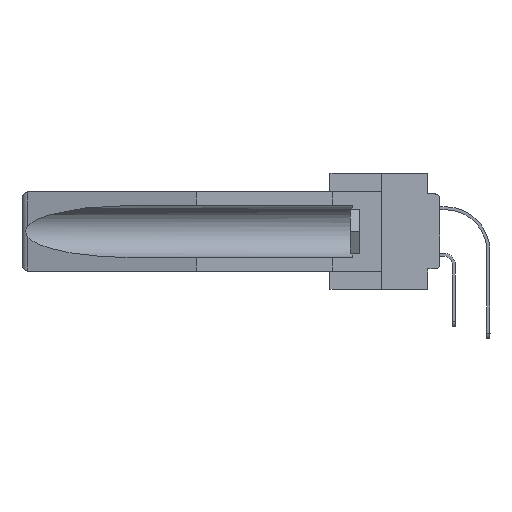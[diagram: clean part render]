
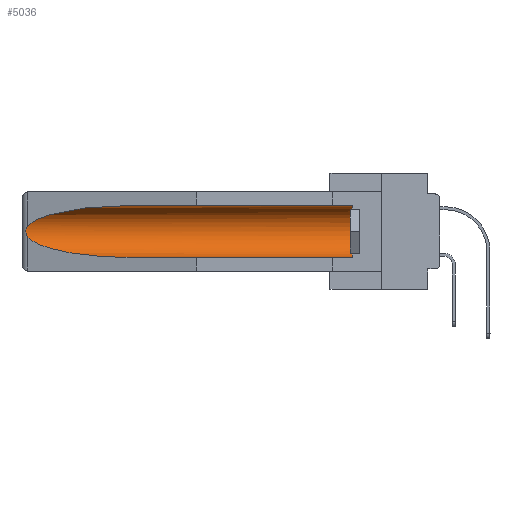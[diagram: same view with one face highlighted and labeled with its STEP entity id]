
A CAD part, left-side view. The second image highlights one B-rep face of the part: STEP entity #5036.
In plain terms, the highlighted cylindrical face has radius 2.857 mm (diameter 5.715 mm), a partial arc.
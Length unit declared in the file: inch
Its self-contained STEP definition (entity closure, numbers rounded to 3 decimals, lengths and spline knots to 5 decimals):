
#527 = CIRCLE ( 'NONE', #28919, 0.1125 ) ;
#611 = EDGE_CURVE ( 'NONE', #28148, #28054, #527, .T. ) ;
#963 = FACE_OUTER_BOUND ( 'NONE', #2200, .T. ) ;
#1455 = CARTESIAN_POINT ( 'NONE',  ( 0.2673, 1.53269, -0.17917 ) ) ;
#1948 = LINE ( 'NONE', #7681, #22371 ) ;
#2200 = EDGE_LOOP ( 'NONE', ( #30819, #31581, #6499, #9714, #12479, #3039 ) ) ;
#2549 = CARTESIAN_POINT ( 'NONE',  ( 0.26537, 1.52718, -0.19328 ) ) ;
#2904 = CARTESIAN_POINT ( 'NONE',  ( 0.25451, 1.48313, -0.09465 ) ) ;
#3039 = ORIENTED_EDGE ( 'NONE', *, *, #29649, .T. ) ;
#4107 = CARTESIAN_POINT ( 'NONE',  ( 0.155, 0.126, -0.284 ) ) ;
#4379 = VERTEX_POINT ( 'NONE', #20845 ) ;
#4663 = CARTESIAN_POINT ( 'NONE',  ( 0.155, 0.126, -0.059 ) ) ;
#5036 = ADVANCED_FACE ( 'NONE', ( #963 ), #13415, .F. ) ;
#5445 = CARTESIAN_POINT ( 'NONE',  ( 0.26537, 1.52718, -0.19328 ) ) ;
#5510 = CARTESIAN_POINT ( 'NONE',  ( 0.155, 1.07973, -0.059 ) ) ;
#5533 = CARTESIAN_POINT ( 'NONE',  ( 0.25451, 1.48313, -0.24835 ) ) ;
#6499 = ORIENTED_EDGE ( 'NONE', *, *, #9204, .T. ) ;
#7393 = CARTESIAN_POINT ( 'NONE',  ( 0.2675, 1.53308, -0.16763 ) ) ;
#7681 = CARTESIAN_POINT ( 'NONE',  ( 0.155, -0.30754, -0.284 ) ) ;
#9204 = EDGE_CURVE ( 'NONE', #37870, #4379, #16370, .T. ) ;
#9714 = ORIENTED_EDGE ( 'NONE', *, *, #23335, .F. ) ;
#10958 = CARTESIAN_POINT ( 'NONE',  ( 0.26537, 1.52718, -0.14972 ) ) ;
#12479 = ORIENTED_EDGE ( 'NONE', *, *, #611, .T. ) ;
#12557 = CARTESIAN_POINT ( 'NONE',  ( 0.26537, 1.52718, -0.14972 ) ) ;
#13068 = EDGE_CURVE ( 'NONE', #22084, #29655, #28942, .T. ) ;
#13267 = B_SPLINE_CURVE_WITH_KNOTS ( 'NONE', 3,
 ( #10958, #34400, #31852, #25753, #7393, #16682, #1455, #28706, #31441, #16884 ),
 .UNSPECIFIED., .F., .F.,
 ( 4, 2, 2, 2, 4 ),
 ( 0., 0.00029, 0.00058, 0.00087, 0.00117 ),
 .UNSPECIFIED. ) ;
#13415 = CYLINDRICAL_SURFACE ( 'NONE', #13519, 0.1125 ) ;
#13519 = AXIS2_PLACEMENT_3D ( 'NONE', #15779, #34482, #25453 ) ;
#15353 = VECTOR ( 'NONE', #37821, 39.37008 ) ;
#15779 = CARTESIAN_POINT ( 'NONE',  ( 0.155, -0.30754, -0.1715 ) ) ;
#16370 =( BOUNDED_CURVE ( )  B_SPLINE_CURVE ( 3, ( #2549, #5533, #17577, #27567 ),
 .UNSPECIFIED., .F., .F. ) 
 B_SPLINE_CURVE_WITH_KNOTS ( ( 4, 4 ),
 ( 0.1948, 1.5708 ),
 .UNSPECIFIED. ) 
 CURVE ( )  GEOMETRIC_REPRESENTATION_ITEM ( )  RATIONAL_B_SPLINE_CURVE ( ( 1., 0.848, 0.848, 1. ) ) 
 REPRESENTATION_ITEM ( '' )  );
#16682 = CARTESIAN_POINT ( 'NONE',  ( 0.2675, 1.53308, -0.17534 ) ) ;
#16884 = CARTESIAN_POINT ( 'NONE',  ( 0.26537, 1.52718, -0.19328 ) ) ;
#16955 = LINE ( 'NONE', #23076, #15353 ) ;
#17577 = CARTESIAN_POINT ( 'NONE',  ( 0.21114, 1.30732, -0.284 ) ) ;
#19797 = EDGE_CURVE ( 'NONE', #29655, #37870, #13267, .T. ) ;
#19952 = DIRECTION ( 'NONE',  ( 0., 1., 0. ) ) ;
#20845 = CARTESIAN_POINT ( 'NONE',  ( 0.155, 1.07973, -0.284 ) ) ;
#22084 = VERTEX_POINT ( 'NONE', #5510 ) ;
#22371 = VECTOR ( 'NONE', #19952, 39.37008 ) ;
#23076 = CARTESIAN_POINT ( 'NONE',  ( 0.155, -0.30754, -0.059 ) ) ;
#23335 = EDGE_CURVE ( 'NONE', #28148, #4379, #1948, .T. ) ;
#24017 = DIRECTION ( 'NONE',  ( 0., 0., 1. ) ) ;
#25453 = DIRECTION ( 'NONE',  ( 0., 0., 1. ) ) ;
#25753 = CARTESIAN_POINT ( 'NONE',  ( 0.2673, 1.5327, -0.16383 ) ) ;
#26979 = CARTESIAN_POINT ( 'NONE',  ( 0.155, 0.126, -0.1715 ) ) ;
#27557 = CARTESIAN_POINT ( 'NONE',  ( 0.21114, 1.30732, -0.059 ) ) ;
#27567 = CARTESIAN_POINT ( 'NONE',  ( 0.155, 1.07973, -0.284 ) ) ;
#28054 = VERTEX_POINT ( 'NONE', #4663 ) ;
#28148 = VERTEX_POINT ( 'NONE', #4107 ) ;
#28706 = CARTESIAN_POINT ( 'NONE',  ( 0.26655, 1.53094, -0.18657 ) ) ;
#28919 = AXIS2_PLACEMENT_3D ( 'NONE', #26979, #38973, #24017 ) ;
#28942 =( BOUNDED_CURVE ( )  B_SPLINE_CURVE ( 3, ( #36406, #27557, #2904, #12557 ),
 .UNSPECIFIED., .F., .F. ) 
 B_SPLINE_CURVE_WITH_KNOTS ( ( 4, 4 ),
 ( 4.71239, 6.08839 ),
 .UNSPECIFIED. ) 
 CURVE ( )  GEOMETRIC_REPRESENTATION_ITEM ( )  RATIONAL_B_SPLINE_CURVE ( ( 1., 0.848, 0.848, 1. ) ) 
 REPRESENTATION_ITEM ( '' )  );
#29649 = EDGE_CURVE ( 'NONE', #28054, #22084, #16955, .T. ) ;
#29655 = VERTEX_POINT ( 'NONE', #38026 ) ;
#30819 = ORIENTED_EDGE ( 'NONE', *, *, #13068, .T. ) ;
#31441 = CARTESIAN_POINT ( 'NONE',  ( 0.26597, 1.5296, -0.19026 ) ) ;
#31581 = ORIENTED_EDGE ( 'NONE', *, *, #19797, .T. ) ;
#31852 = CARTESIAN_POINT ( 'NONE',  ( 0.26654, 1.53092, -0.15636 ) ) ;
#34400 = CARTESIAN_POINT ( 'NONE',  ( 0.26597, 1.52961, -0.15275 ) ) ;
#34482 = DIRECTION ( 'NONE',  ( 0., 1., 0. ) ) ;
#36406 = CARTESIAN_POINT ( 'NONE',  ( 0.155, 1.07973, -0.059 ) ) ;
#37821 = DIRECTION ( 'NONE',  ( 0., 1., 0. ) ) ;
#37870 = VERTEX_POINT ( 'NONE', #5445 ) ;
#38026 = CARTESIAN_POINT ( 'NONE',  ( 0.26537, 1.52718, -0.14972 ) ) ;
#38973 = DIRECTION ( 'NONE',  ( 0., -1., 0. ) ) ;
